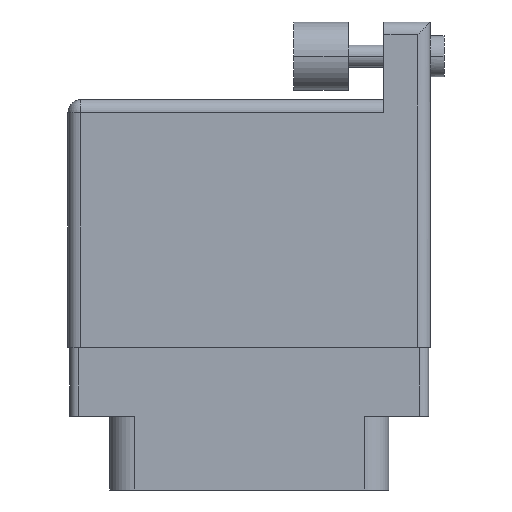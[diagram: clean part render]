
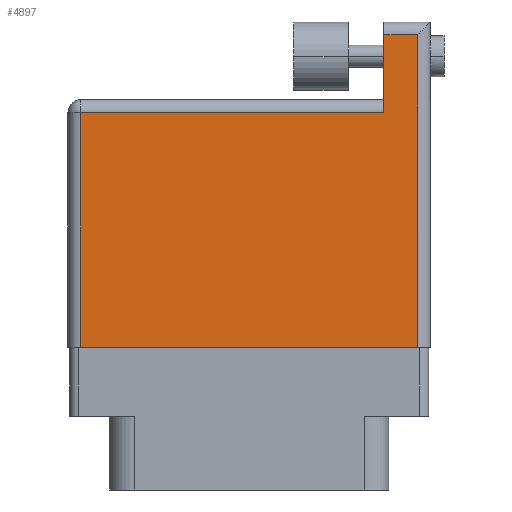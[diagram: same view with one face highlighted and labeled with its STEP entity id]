
A CAD part, front view. The second image highlights one B-rep face of the part: STEP entity #4897.
In plain terms, the highlighted face is planar.
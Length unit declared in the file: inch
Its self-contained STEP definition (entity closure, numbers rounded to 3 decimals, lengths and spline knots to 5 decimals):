
#705 = LINE ( 'NONE', #17621, #24957 ) ;
#888 = VERTEX_POINT ( 'NONE', #1511 ) ;
#1511 = CARTESIAN_POINT ( 'NONE',  ( 1.155, 1.143, 0. ) ) ;
#1816 = CARTESIAN_POINT ( 'NONE',  ( 0., 0.859, 0. ) ) ;
#2889 = LINE ( 'NONE', #1816, #22041 ) ;
#4255 = DIRECTION ( 'NONE',  ( 0., -1., 0. ) ) ;
#4561 = DIRECTION ( 'NONE',  ( -1., 0., 0. ) ) ;
#4897 = ADVANCED_FACE ( 'NONE', ( #20089 ), #6684, .F. ) ;
#5208 = LINE ( 'NONE', #20461, #23390 ) ;
#5339 = AXIS2_PLACEMENT_3D ( 'NONE', #23096, #24874, #4561 ) ;
#5759 = LINE ( 'NONE', #20501, #23313 ) ;
#5907 = LINE ( 'NONE', #8786, #21259 ) ;
#6390 = ORIENTED_EDGE ( 'NONE', *, *, #21839, .T. ) ;
#6517 = LINE ( 'NONE', #25420, #8434 ) ;
#6684 = PLANE ( 'NONE',  #5339 ) ;
#6888 = EDGE_CURVE ( 'NONE', #17709, #10367, #5907, .T. ) ;
#7615 = DIRECTION ( 'NONE',  ( -1., 0., 0. ) ) ;
#7703 = ORIENTED_EDGE ( 'NONE', *, *, #16815, .T. ) ;
#8434 = VECTOR ( 'NONE', #17175, 39.37008 ) ;
#8786 = CARTESIAN_POINT ( 'NONE',  ( 0.047, 0., 0. ) ) ;
#9567 = CARTESIAN_POINT ( 'NONE',  ( 1.155, 0.859, 0. ) ) ;
#10367 = VERTEX_POINT ( 'NONE', #25352 ) ;
#10855 = DIRECTION ( 'NONE',  ( 0., -1., 0. ) ) ;
#11189 = ORIENTED_EDGE ( 'NONE', *, *, #15170, .T. ) ;
#12187 = VERTEX_POINT ( 'NONE', #14835 ) ;
#13433 = EDGE_CURVE ( 'NONE', #16044, #888, #5208, .T. ) ;
#14835 = CARTESIAN_POINT ( 'NONE',  ( 1.278, 0., 0. ) ) ;
#15170 = EDGE_CURVE ( 'NONE', #10367, #12187, #705, .T. ) ;
#16044 = VERTEX_POINT ( 'NONE', #22278 ) ;
#16047 = ORIENTED_EDGE ( 'NONE', *, *, #16658, .T. ) ;
#16658 = EDGE_CURVE ( 'NONE', #17738, #17709, #2889, .T. ) ;
#16815 = EDGE_CURVE ( 'NONE', #888, #17738, #5759, .T. ) ;
#17175 = DIRECTION ( 'NONE',  ( 0., 1., 0. ) ) ;
#17621 = CARTESIAN_POINT ( 'NONE',  ( 0., 0., 0. ) ) ;
#17709 = VERTEX_POINT ( 'NONE', #23730 ) ;
#17738 = VERTEX_POINT ( 'NONE', #9567 ) ;
#17805 = ORIENTED_EDGE ( 'NONE', *, *, #13433, .T. ) ;
#18626 = EDGE_LOOP ( 'NONE', ( #11189, #6390, #17805, #7703, #16047, #19263 ) ) ;
#19263 = ORIENTED_EDGE ( 'NONE', *, *, #6888, .T. ) ;
#20089 = FACE_OUTER_BOUND ( 'NONE', #18626, .T. ) ;
#20461 = CARTESIAN_POINT ( 'NONE',  ( 1.155, 1.143, 0. ) ) ;
#20501 = CARTESIAN_POINT ( 'NONE',  ( 1.155, 1.19, 0. ) ) ;
#21257 = DIRECTION ( 'NONE',  ( 1., 0., 0. ) ) ;
#21259 = VECTOR ( 'NONE', #10855, 39.37008 ) ;
#21839 = EDGE_CURVE ( 'NONE', #12187, #16044, #6517, .T. ) ;
#22041 = VECTOR ( 'NONE', #7615, 39.37008 ) ;
#22278 = CARTESIAN_POINT ( 'NONE',  ( 1.278, 1.143, 0. ) ) ;
#23096 = CARTESIAN_POINT ( 'NONE',  ( 0., 0.906, 0. ) ) ;
#23313 = VECTOR ( 'NONE', #4255, 39.37008 ) ;
#23390 = VECTOR ( 'NONE', #24611, 39.37008 ) ;
#23730 = CARTESIAN_POINT ( 'NONE',  ( 0.047, 0.859, 0. ) ) ;
#24611 = DIRECTION ( 'NONE',  ( -1., 0., 0. ) ) ;
#24874 = DIRECTION ( 'NONE',  ( 0., 0., -1. ) ) ;
#24957 = VECTOR ( 'NONE', #21257, 39.37008 ) ;
#25352 = CARTESIAN_POINT ( 'NONE',  ( 0.047, 0., 0. ) ) ;
#25420 = CARTESIAN_POINT ( 'NONE',  ( 1.278, 1.19, 0. ) ) ;
